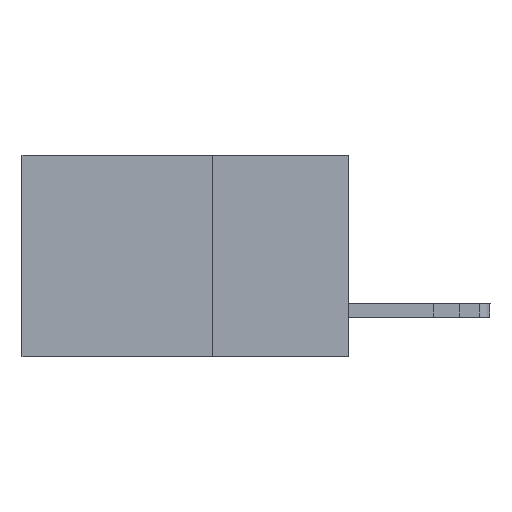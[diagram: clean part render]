
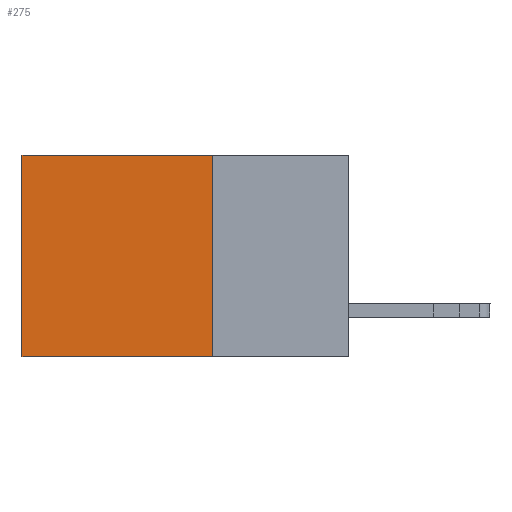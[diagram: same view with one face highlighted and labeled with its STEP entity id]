
A CAD part, left-side view. The second image highlights one B-rep face of the part: STEP entity #275.
In plain terms, the highlighted planar face has unit normal (-1, 0, 0).
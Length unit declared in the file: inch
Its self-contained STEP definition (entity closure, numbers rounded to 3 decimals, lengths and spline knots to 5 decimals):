
#117 = CARTESIAN_POINT ( 'NONE',  ( 0.2615, 0.25, 0. ) ) ;
#124 = DIRECTION ( 'NONE',  ( 1., 0., 0. ) ) ;
#206 = DIRECTION ( 'NONE',  ( 0., 0., -1. ) ) ;
#275 = ADVANCED_FACE ( 'NONE', ( #8290 ), #2314, .F. ) ;
#709 = DIRECTION ( 'NONE',  ( 0., 0., -1. ) ) ;
#967 = DIRECTION ( 'NONE',  ( 0., 0., -1. ) ) ;
#1416 = VECTOR ( 'NONE', #6738, 39.37008 ) ;
#1710 = EDGE_CURVE ( 'NONE', #15405, #11271, #4097, .T. ) ;
#1938 = CARTESIAN_POINT ( 'NONE',  ( 0.2615, 0.25, 0. ) ) ;
#1965 = ORIENTED_EDGE ( 'NONE', *, *, #1710, .F. ) ;
#2314 = PLANE ( 'NONE',  #10113 ) ;
#3069 = CARTESIAN_POINT ( 'NONE',  ( 0.2615, 0.25, -0.37 ) ) ;
#3081 = CARTESIAN_POINT ( 'NONE',  ( 0.2615, 0.25, -0.37 ) ) ;
#4097 = LINE ( 'NONE', #3081, #13516 ) ;
#4180 = DIRECTION ( 'NONE',  ( 0., 1., 0. ) ) ;
#4695 = EDGE_CURVE ( 'NONE', #14563, #11271, #7852, .T. ) ;
#4747 = CARTESIAN_POINT ( 'NONE',  ( 0.2615, 0.25, -0.37 ) ) ;
#6337 = CARTESIAN_POINT ( 'NONE',  ( 0.2615, 0.6, 0. ) ) ;
#6738 = DIRECTION ( 'NONE',  ( 0., 1., 0. ) ) ;
#6744 = CARTESIAN_POINT ( 'NONE',  ( 0.2615, 0.6, -0.37 ) ) ;
#7852 = LINE ( 'NONE', #6744, #13839 ) ;
#7925 = LINE ( 'NONE', #1938, #1416 ) ;
#8283 = ORIENTED_EDGE ( 'NONE', *, *, #9387, .F. ) ;
#8290 = FACE_OUTER_BOUND ( 'NONE', #8353, .T. ) ;
#8353 = EDGE_LOOP ( 'NONE', ( #10613, #1965, #8283, #11485 ) ) ;
#9265 = CARTESIAN_POINT ( 'NONE',  ( 0.2615, 0.6, -0.37 ) ) ;
#9387 = EDGE_CURVE ( 'NONE', #10464, #15405, #11626, .T. ) ;
#10113 = AXIS2_PLACEMENT_3D ( 'NONE', #13063, #124, #206 ) ;
#10464 = VERTEX_POINT ( 'NONE', #117 ) ;
#10613 = ORIENTED_EDGE ( 'NONE', *, *, #4695, .T. ) ;
#11271 = VERTEX_POINT ( 'NONE', #9265 ) ;
#11485 = ORIENTED_EDGE ( 'NONE', *, *, #13515, .T. ) ;
#11626 = LINE ( 'NONE', #3069, #13420 ) ;
#13063 = CARTESIAN_POINT ( 'NONE',  ( 0.2615, 0.25, -0.37 ) ) ;
#13420 = VECTOR ( 'NONE', #967, 39.37008 ) ;
#13515 = EDGE_CURVE ( 'NONE', #10464, #14563, #7925, .T. ) ;
#13516 = VECTOR ( 'NONE', #4180, 39.37008 ) ;
#13839 = VECTOR ( 'NONE', #709, 39.37008 ) ;
#14563 = VERTEX_POINT ( 'NONE', #6337 ) ;
#15405 = VERTEX_POINT ( 'NONE', #4747 ) ;
